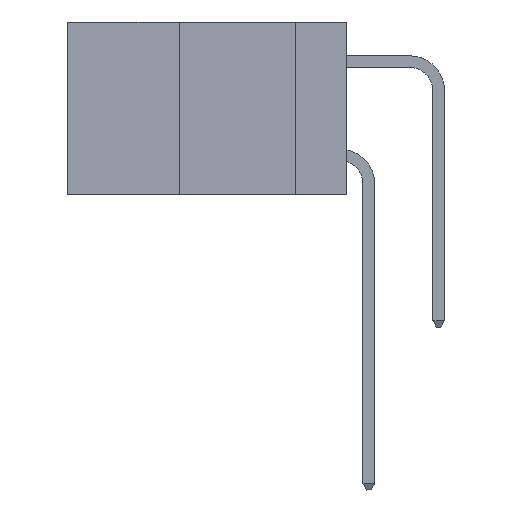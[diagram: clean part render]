
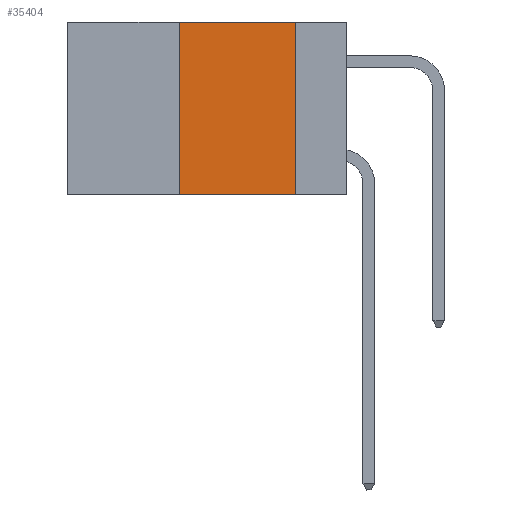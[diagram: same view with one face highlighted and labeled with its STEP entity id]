
A CAD part, left-side view. The second image highlights one B-rep face of the part: STEP entity #35404.
In plain terms, the highlighted planar face has unit normal (-1, 0, 0).
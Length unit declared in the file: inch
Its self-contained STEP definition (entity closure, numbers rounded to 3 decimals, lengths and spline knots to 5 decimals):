
#1910 = VERTEX_POINT ( 'NONE', #35612 ) ;
#2889 = ORIENTED_EDGE ( 'NONE', *, *, #19051, .F. ) ;
#5321 = CARTESIAN_POINT ( 'NONE',  ( 0., 0.6, 0. ) ) ;
#6547 = CARTESIAN_POINT ( 'NONE',  ( 0., 0.36, 0. ) ) ;
#6856 = CARTESIAN_POINT ( 'NONE',  ( 0., 0.36, 0. ) ) ;
#7336 = PLANE ( 'NONE',  #24336 ) ;
#8926 = VERTEX_POINT ( 'NONE', #15175 ) ;
#10123 = CARTESIAN_POINT ( 'NONE',  ( 0., 0.11, 0. ) ) ;
#13087 = VERTEX_POINT ( 'NONE', #23893 ) ;
#13948 = VECTOR ( 'NONE', #40618, 39.37008 ) ;
#14307 = ORIENTED_EDGE ( 'NONE', *, *, #31847, .T. ) ;
#15175 = CARTESIAN_POINT ( 'NONE',  ( 0., 0.36, -0.37 ) ) ;
#16853 = VECTOR ( 'NONE', #17929, 39.37008 ) ;
#17243 = LINE ( 'NONE', #6856, #16853 ) ;
#17496 = FACE_OUTER_BOUND ( 'NONE', #36993, .T. ) ;
#17929 = DIRECTION ( 'NONE',  ( 0., 0., 1. ) ) ;
#19051 = EDGE_CURVE ( 'NONE', #8926, #36315, #17243, .T. ) ;
#19664 = CARTESIAN_POINT ( 'NONE',  ( 0., 0.6, -0.37 ) ) ;
#21410 = DIRECTION ( 'NONE',  ( 1., 0., 0. ) ) ;
#23893 = CARTESIAN_POINT ( 'NONE',  ( 0., 0.11, 0. ) ) ;
#24336 = AXIS2_PLACEMENT_3D ( 'NONE', #27870, #21410, #28322 ) ;
#25905 = ORIENTED_EDGE ( 'NONE', *, *, #43157, .F. ) ;
#27828 = VECTOR ( 'NONE', #31105, 39.37008 ) ;
#27870 = CARTESIAN_POINT ( 'NONE',  ( 0., 0.6, 0. ) ) ;
#28322 = DIRECTION ( 'NONE',  ( 0., 0., -1. ) ) ;
#28729 = ORIENTED_EDGE ( 'NONE', *, *, #33669, .F. ) ;
#30267 = DIRECTION ( 'NONE',  ( 0., -1., 0. ) ) ;
#30648 = LINE ( 'NONE', #10123, #27828 ) ;
#31105 = DIRECTION ( 'NONE',  ( 0., 0., -1. ) ) ;
#31847 = EDGE_CURVE ( 'NONE', #8926, #1910, #44365, .T. ) ;
#33669 = EDGE_CURVE ( 'NONE', #36315, #13087, #43851, .T. ) ;
#35404 = ADVANCED_FACE ( 'NONE', ( #17496 ), #7336, .F. ) ;
#35612 = CARTESIAN_POINT ( 'NONE',  ( 0., 0.11, -0.37 ) ) ;
#36315 = VERTEX_POINT ( 'NONE', #6547 ) ;
#36993 = EDGE_LOOP ( 'NONE', ( #25905, #28729, #2889, #14307 ) ) ;
#40618 = DIRECTION ( 'NONE',  ( 0., -1., 0. ) ) ;
#43157 = EDGE_CURVE ( 'NONE', #13087, #1910, #30648, .T. ) ;
#43851 = LINE ( 'NONE', #5321, #13948 ) ;
#44048 = VECTOR ( 'NONE', #30267, 39.37008 ) ;
#44365 = LINE ( 'NONE', #19664, #44048 ) ;
